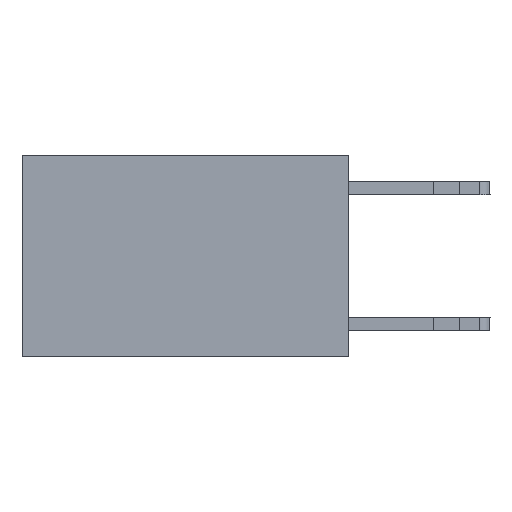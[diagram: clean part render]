
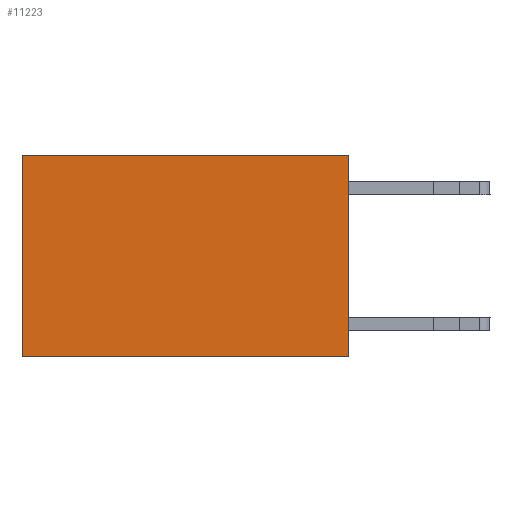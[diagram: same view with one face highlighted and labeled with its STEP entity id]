
A CAD part, left-side view. The second image highlights one B-rep face of the part: STEP entity #11223.
In plain terms, the highlighted planar face has unit normal (-1, 0, 0).
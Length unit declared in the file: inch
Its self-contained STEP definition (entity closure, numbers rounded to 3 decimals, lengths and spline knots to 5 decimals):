
#477 = LINE ( 'NONE', #9128, #12530 ) ;
#490 = EDGE_CURVE ( 'NONE', #13423, #13702, #13357, .T. ) ;
#742 = ORIENTED_EDGE ( 'NONE', *, *, #13917, .T. ) ;
#940 = CARTESIAN_POINT ( 'NONE',  ( 0.2625, 0., 0. ) ) ;
#1118 = CARTESIAN_POINT ( 'NONE',  ( 0.2625, 0., -0.37 ) ) ;
#2170 = CARTESIAN_POINT ( 'NONE',  ( 0.2625, 0., 0. ) ) ;
#2443 = VECTOR ( 'NONE', #8585, 39.37008 ) ;
#2561 = VECTOR ( 'NONE', #7889, 39.37008 ) ;
#3532 = CARTESIAN_POINT ( 'NONE',  ( 0.2625, 0., 0. ) ) ;
#4534 = DIRECTION ( 'NONE',  ( 0., 0., -1. ) ) ;
#5136 = ORIENTED_EDGE ( 'NONE', *, *, #490, .F. ) ;
#6114 = DIRECTION ( 'NONE',  ( 1., 0., 0. ) ) ;
#6685 = EDGE_CURVE ( 'NONE', #13702, #11471, #7822, .T. ) ;
#7822 = LINE ( 'NONE', #1118, #2561 ) ;
#7889 = DIRECTION ( 'NONE',  ( 0., 1., 0. ) ) ;
#8254 = DIRECTION ( 'NONE',  ( 0., 0., -1. ) ) ;
#8283 = DIRECTION ( 'NONE',  ( 0., 0., -1. ) ) ;
#8585 = DIRECTION ( 'NONE',  ( 0., 1., 0. ) ) ;
#9128 = CARTESIAN_POINT ( 'NONE',  ( 0.2625, 0.6, 0. ) ) ;
#9293 = FACE_OUTER_BOUND ( 'NONE', #12821, .T. ) ;
#9414 = CARTESIAN_POINT ( 'NONE',  ( 0.2625, 0., -0.37 ) ) ;
#10040 = LINE ( 'NONE', #2170, #2443 ) ;
#10694 = VECTOR ( 'NONE', #8283, 39.37008 ) ;
#10978 = ORIENTED_EDGE ( 'NONE', *, *, #14030, .T. ) ;
#11083 = AXIS2_PLACEMENT_3D ( 'NONE', #13665, #6114, #8254 ) ;
#11140 = CARTESIAN_POINT ( 'NONE',  ( 0.2625, 0.6, -0.37 ) ) ;
#11223 = ADVANCED_FACE ( 'NONE', ( #9293 ), #11449, .F. ) ;
#11449 = PLANE ( 'NONE',  #11083 ) ;
#11471 = VERTEX_POINT ( 'NONE', #11140 ) ;
#11924 = VERTEX_POINT ( 'NONE', #12750 ) ;
#12530 = VECTOR ( 'NONE', #4534, 39.37008 ) ;
#12750 = CARTESIAN_POINT ( 'NONE',  ( 0.2625, 0.6, 0. ) ) ;
#12821 = EDGE_LOOP ( 'NONE', ( #10978, #13101, #5136, #742 ) ) ;
#13101 = ORIENTED_EDGE ( 'NONE', *, *, #6685, .F. ) ;
#13357 = LINE ( 'NONE', #3532, #10694 ) ;
#13423 = VERTEX_POINT ( 'NONE', #940 ) ;
#13665 = CARTESIAN_POINT ( 'NONE',  ( 0.2625, 0., 0. ) ) ;
#13702 = VERTEX_POINT ( 'NONE', #9414 ) ;
#13917 = EDGE_CURVE ( 'NONE', #13423, #11924, #10040, .T. ) ;
#14030 = EDGE_CURVE ( 'NONE', #11924, #11471, #477, .T. ) ;
